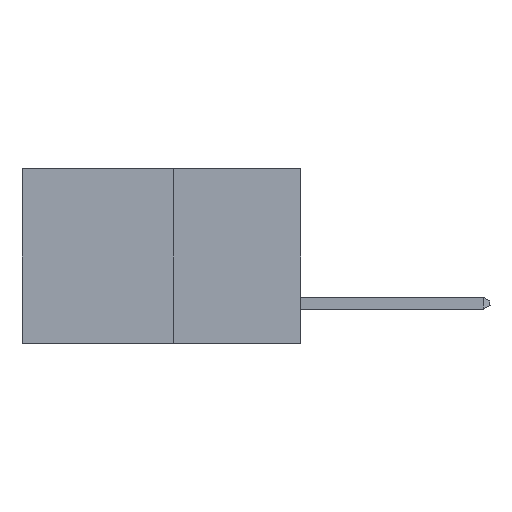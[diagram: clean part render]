
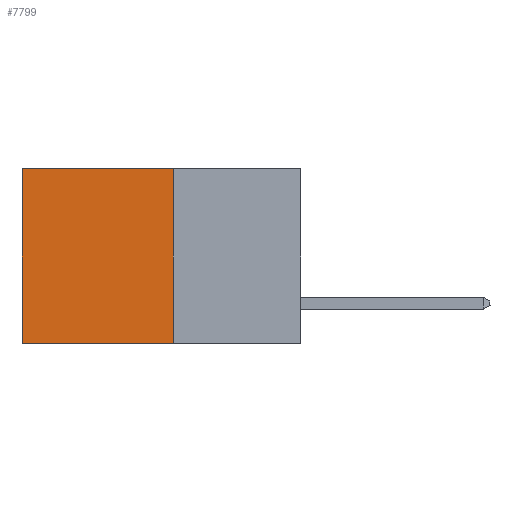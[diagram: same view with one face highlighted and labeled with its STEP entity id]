
A CAD part, left-side view. The second image highlights one B-rep face of the part: STEP entity #7799.
In plain terms, the highlighted planar face has unit normal (-1, 0, 0).
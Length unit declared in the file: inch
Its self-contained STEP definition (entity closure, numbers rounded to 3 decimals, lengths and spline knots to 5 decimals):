
#287 = VECTOR ( 'NONE', #17681, 39.37008 ) ;
#299 = EDGE_LOOP ( 'NONE', ( #17544, #13717, #1635, #8837 ) ) ;
#461 = VERTEX_POINT ( 'NONE', #9173 ) ;
#1635 = ORIENTED_EDGE ( 'NONE', *, *, #4239, .F. ) ;
#3411 = CARTESIAN_POINT ( 'NONE',  ( 0.277, 0.27, 0. ) ) ;
#4239 = EDGE_CURVE ( 'NONE', #5471, #4613, #15177, .T. ) ;
#4613 = VERTEX_POINT ( 'NONE', #12857 ) ;
#4681 = LINE ( 'NONE', #9740, #8698 ) ;
#5471 = VERTEX_POINT ( 'NONE', #3411 ) ;
#5594 = VECTOR ( 'NONE', #16355, 39.37008 ) ;
#6044 = VERTEX_POINT ( 'NONE', #15855 ) ;
#6232 = DIRECTION ( 'NONE',  ( 0., 0., -1. ) ) ;
#7799 = ADVANCED_FACE ( 'NONE', ( #18236 ), #10718, .F. ) ;
#7881 = CARTESIAN_POINT ( 'NONE',  ( 0.277, 0.27, -0.37 ) ) ;
#8698 = VECTOR ( 'NONE', #6232, 39.37008 ) ;
#8837 = ORIENTED_EDGE ( 'NONE', *, *, #14529, .T. ) ;
#9104 = AXIS2_PLACEMENT_3D ( 'NONE', #10547, #10526, #10501 ) ;
#9173 = CARTESIAN_POINT ( 'NONE',  ( 0.277, 0.59, 0. ) ) ;
#9740 = CARTESIAN_POINT ( 'NONE',  ( 0.277, 0.59, -0.37 ) ) ;
#10501 = DIRECTION ( 'NONE',  ( 0., 0., -1. ) ) ;
#10526 = DIRECTION ( 'NONE',  ( 1., 0., 0. ) ) ;
#10547 = CARTESIAN_POINT ( 'NONE',  ( 0.277, 0.27, -0.37 ) ) ;
#10718 = PLANE ( 'NONE',  #9104 ) ;
#12157 = LINE ( 'NONE', #7881, #20495 ) ;
#12857 = CARTESIAN_POINT ( 'NONE',  ( 0.277, 0.27, -0.37 ) ) ;
#13717 = ORIENTED_EDGE ( 'NONE', *, *, #21308, .F. ) ;
#13963 = LINE ( 'NONE', #16019, #287 ) ;
#14529 = EDGE_CURVE ( 'NONE', #5471, #461, #13963, .T. ) ;
#15177 = LINE ( 'NONE', #16433, #5594 ) ;
#15855 = CARTESIAN_POINT ( 'NONE',  ( 0.277, 0.59, -0.37 ) ) ;
#16019 = CARTESIAN_POINT ( 'NONE',  ( 0.277, 0.27, 0. ) ) ;
#16355 = DIRECTION ( 'NONE',  ( 0., 0., -1. ) ) ;
#16433 = CARTESIAN_POINT ( 'NONE',  ( 0.277, 0.27, -0.37 ) ) ;
#17544 = ORIENTED_EDGE ( 'NONE', *, *, #20842, .T. ) ;
#17681 = DIRECTION ( 'NONE',  ( 0., 1., 0. ) ) ;
#18236 = FACE_OUTER_BOUND ( 'NONE', #299, .T. ) ;
#19677 = DIRECTION ( 'NONE',  ( 0., 1., 0. ) ) ;
#20495 = VECTOR ( 'NONE', #19677, 39.37008 ) ;
#20842 = EDGE_CURVE ( 'NONE', #461, #6044, #4681, .T. ) ;
#21308 = EDGE_CURVE ( 'NONE', #4613, #6044, #12157, .T. ) ;
